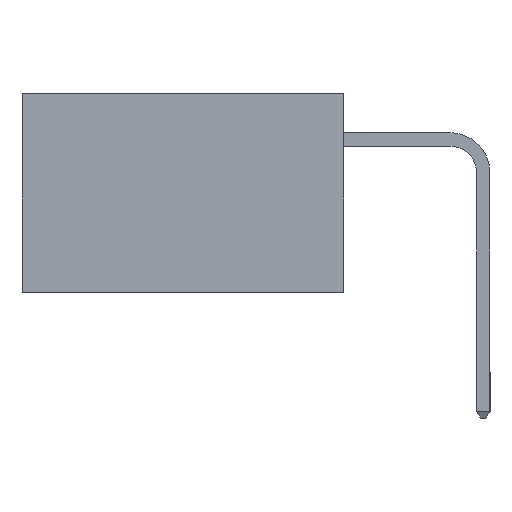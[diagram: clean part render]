
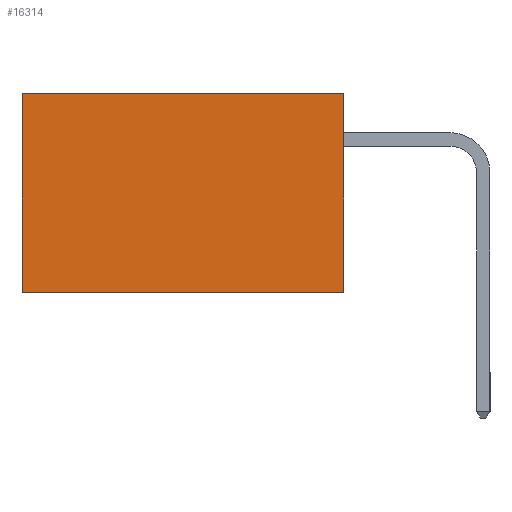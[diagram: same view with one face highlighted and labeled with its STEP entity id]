
A CAD part, left-side view. The second image highlights one B-rep face of the part: STEP entity #16314.
In plain terms, the highlighted planar face has unit normal (-1, 0, 0).
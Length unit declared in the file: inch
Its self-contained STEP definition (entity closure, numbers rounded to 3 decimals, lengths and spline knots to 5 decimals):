
#652 = DIRECTION ( 'NONE',  ( 0., 1., 0. ) ) ;
#1170 = CARTESIAN_POINT ( 'NONE',  ( 0.298, 0., 0. ) ) ;
#2409 = VERTEX_POINT ( 'NONE', #8841 ) ;
#3266 = CARTESIAN_POINT ( 'NONE',  ( 0.298, 0., 0. ) ) ;
#3814 = PLANE ( 'NONE',  #24532 ) ;
#4760 = CARTESIAN_POINT ( 'NONE',  ( 0.298, 0., -0.37 ) ) ;
#6928 = VECTOR ( 'NONE', #7387, 39.37008 ) ;
#7226 = ORIENTED_EDGE ( 'NONE', *, *, #7424, .F. ) ;
#7271 = CARTESIAN_POINT ( 'NONE',  ( 0.298, 0., 0. ) ) ;
#7387 = DIRECTION ( 'NONE',  ( 0., 1., 0. ) ) ;
#7408 = ORIENTED_EDGE ( 'NONE', *, *, #20806, .T. ) ;
#7424 = EDGE_CURVE ( 'NONE', #11306, #11290, #26060, .T. ) ;
#7925 = DIRECTION ( 'NONE',  ( 1., 0., 0. ) ) ;
#8841 = CARTESIAN_POINT ( 'NONE',  ( 0.298, 0.6, 0. ) ) ;
#11290 = VERTEX_POINT ( 'NONE', #20093 ) ;
#11306 = VERTEX_POINT ( 'NONE', #26009 ) ;
#14223 = CARTESIAN_POINT ( 'NONE',  ( 0.298, 0.6, 0. ) ) ;
#14703 = VERTEX_POINT ( 'NONE', #1170 ) ;
#14964 = VECTOR ( 'NONE', #25331, 39.37008 ) ;
#16076 = CARTESIAN_POINT ( 'NONE',  ( 0.298, 0., 0. ) ) ;
#16314 = ADVANCED_FACE ( 'NONE', ( #20533 ), #3814, .F. ) ;
#16592 = EDGE_LOOP ( 'NONE', ( #16902, #7226, #16680, #7408 ) ) ;
#16680 = ORIENTED_EDGE ( 'NONE', *, *, #17995, .F. ) ;
#16902 = ORIENTED_EDGE ( 'NONE', *, *, #19728, .T. ) ;
#17995 = EDGE_CURVE ( 'NONE', #14703, #11306, #20240, .T. ) ;
#18277 = LINE ( 'NONE', #14223, #22890 ) ;
#19625 = VECTOR ( 'NONE', #652, 39.37008 ) ;
#19728 = EDGE_CURVE ( 'NONE', #2409, #11290, #18277, .T. ) ;
#20093 = CARTESIAN_POINT ( 'NONE',  ( 0.298, 0.6, -0.37 ) ) ;
#20240 = LINE ( 'NONE', #7271, #14964 ) ;
#20533 = FACE_OUTER_BOUND ( 'NONE', #16592, .T. ) ;
#20806 = EDGE_CURVE ( 'NONE', #14703, #2409, #23009, .T. ) ;
#22044 = DIRECTION ( 'NONE',  ( 0., 0., -1. ) ) ;
#22890 = VECTOR ( 'NONE', #26110, 39.37008 ) ;
#23009 = LINE ( 'NONE', #3266, #6928 ) ;
#24532 = AXIS2_PLACEMENT_3D ( 'NONE', #16076, #7925, #22044 ) ;
#25331 = DIRECTION ( 'NONE',  ( 0., 0., -1. ) ) ;
#26009 = CARTESIAN_POINT ( 'NONE',  ( 0.298, 0., -0.37 ) ) ;
#26060 = LINE ( 'NONE', #4760, #19625 ) ;
#26110 = DIRECTION ( 'NONE',  ( 0., 0., -1. ) ) ;
